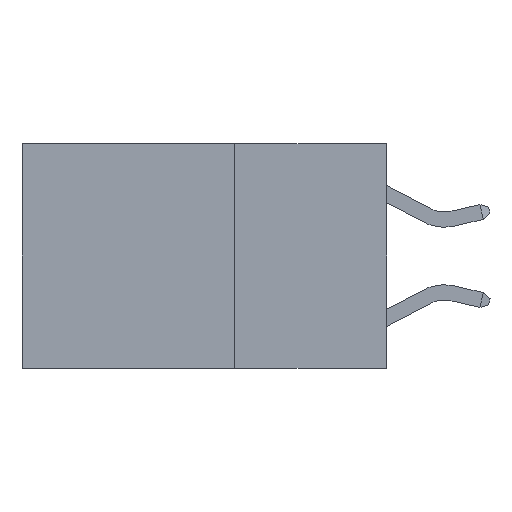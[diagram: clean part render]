
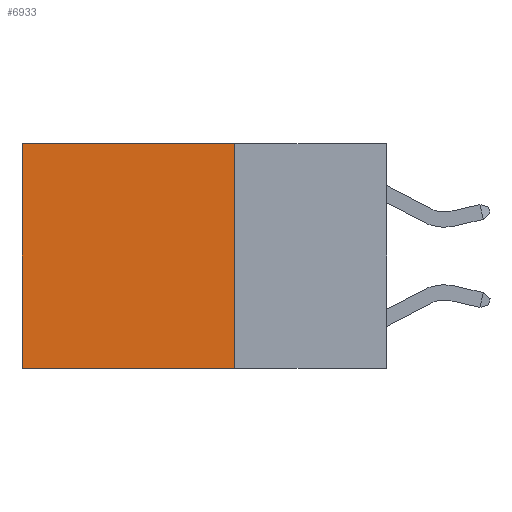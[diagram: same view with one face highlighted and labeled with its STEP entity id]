
A CAD part, left-side view. The second image highlights one B-rep face of the part: STEP entity #6933.
In plain terms, the highlighted planar face has unit normal (-1, 0, 0).
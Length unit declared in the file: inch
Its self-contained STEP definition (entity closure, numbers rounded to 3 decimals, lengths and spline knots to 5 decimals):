
#757 = VECTOR ( 'NONE', #3288, 39.37008 ) ;
#762 = DIRECTION ( 'NONE',  ( 0., 0., -1. ) ) ;
#1459 = VERTEX_POINT ( 'NONE', #26639 ) ;
#2112 = VERTEX_POINT ( 'NONE', #27021 ) ;
#3288 = DIRECTION ( 'NONE',  ( 0., 1., 0. ) ) ;
#3886 = VECTOR ( 'NONE', #16969, 39.37008 ) ;
#4228 = DIRECTION ( 'NONE',  ( 1., 0., 0. ) ) ;
#5084 = CARTESIAN_POINT ( 'NONE',  ( 0.2625, 0.25, 0. ) ) ;
#5535 = CARTESIAN_POINT ( 'NONE',  ( 0.2625, 0.25, 0. ) ) ;
#6782 = ORIENTED_EDGE ( 'NONE', *, *, #14021, .F. ) ;
#6933 = ADVANCED_FACE ( 'NONE', ( #13207 ), #20607, .F. ) ;
#7216 = ORIENTED_EDGE ( 'NONE', *, *, #15535, .T. ) ;
#7273 = EDGE_CURVE ( 'NONE', #24756, #2112, #10614, .T. ) ;
#10136 = LINE ( 'NONE', #5084, #3886 ) ;
#10614 = LINE ( 'NONE', #14800, #28666 ) ;
#13207 = FACE_OUTER_BOUND ( 'NONE', #28324, .T. ) ;
#14021 = EDGE_CURVE ( 'NONE', #1459, #2112, #24255, .T. ) ;
#14216 = VECTOR ( 'NONE', #15672, 39.37008 ) ;
#14800 = CARTESIAN_POINT ( 'NONE',  ( 0.2625, 0.6, 0. ) ) ;
#15535 = EDGE_CURVE ( 'NONE', #16007, #24756, #21964, .T. ) ;
#15672 = DIRECTION ( 'NONE',  ( 0., 1., 0. ) ) ;
#16007 = VERTEX_POINT ( 'NONE', #5535 ) ;
#16969 = DIRECTION ( 'NONE',  ( 0., 0., -1. ) ) ;
#17414 = CARTESIAN_POINT ( 'NONE',  ( 0.2625, 0.25, -0.37 ) ) ;
#18365 = CARTESIAN_POINT ( 'NONE',  ( 0.2625, 0.25, 0. ) ) ;
#18497 = ORIENTED_EDGE ( 'NONE', *, *, #28788, .F. ) ;
#20607 = PLANE ( 'NONE',  #27441 ) ;
#20703 = DIRECTION ( 'NONE',  ( 0., 0., -1. ) ) ;
#21964 = LINE ( 'NONE', #27414, #14216 ) ;
#24255 = LINE ( 'NONE', #17414, #757 ) ;
#24756 = VERTEX_POINT ( 'NONE', #27651 ) ;
#26639 = CARTESIAN_POINT ( 'NONE',  ( 0.2625, 0.25, -0.37 ) ) ;
#27021 = CARTESIAN_POINT ( 'NONE',  ( 0.2625, 0.6, -0.37 ) ) ;
#27414 = CARTESIAN_POINT ( 'NONE',  ( 0.2625, 0.25, 0. ) ) ;
#27441 = AXIS2_PLACEMENT_3D ( 'NONE', #18365, #4228, #20703 ) ;
#27651 = CARTESIAN_POINT ( 'NONE',  ( 0.2625, 0.6, 0. ) ) ;
#28080 = ORIENTED_EDGE ( 'NONE', *, *, #7273, .T. ) ;
#28324 = EDGE_LOOP ( 'NONE', ( #28080, #6782, #18497, #7216 ) ) ;
#28666 = VECTOR ( 'NONE', #762, 39.37008 ) ;
#28788 = EDGE_CURVE ( 'NONE', #16007, #1459, #10136, .T. ) ;
